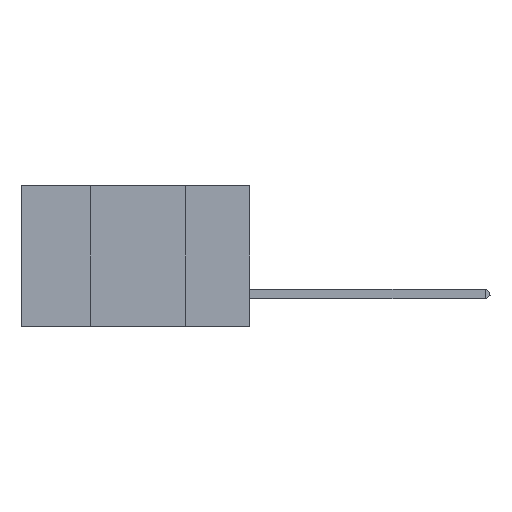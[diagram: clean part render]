
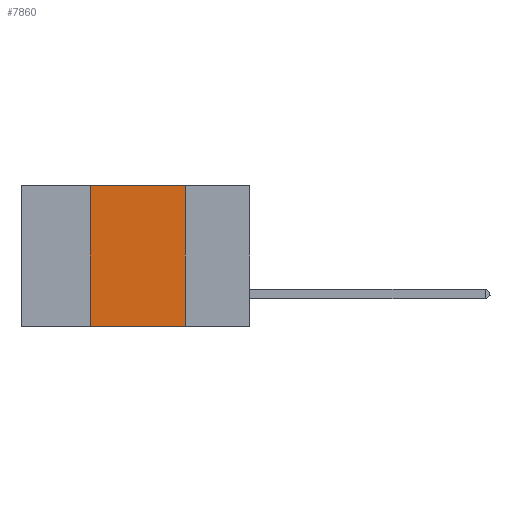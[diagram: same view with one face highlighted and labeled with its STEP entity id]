
A CAD part, left-side view. The second image highlights one B-rep face of the part: STEP entity #7860.
In plain terms, the highlighted planar face has unit normal (-1, 0, 0).
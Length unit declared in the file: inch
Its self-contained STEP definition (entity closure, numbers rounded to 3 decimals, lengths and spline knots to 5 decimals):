
#464 = CARTESIAN_POINT ( 'NONE',  ( 0., 0.42, 0. ) ) ;
#1630 = FACE_OUTER_BOUND ( 'NONE', #16072, .T. ) ;
#1831 = VERTEX_POINT ( 'NONE', #4936 ) ;
#2983 = LINE ( 'NONE', #19520, #17494 ) ;
#3559 = EDGE_CURVE ( 'NONE', #21737, #1831, #23307, .T. ) ;
#3567 = LINE ( 'NONE', #14143, #16220 ) ;
#3700 = DIRECTION ( 'NONE',  ( 0., 0., -1. ) ) ;
#4757 = DIRECTION ( 'NONE',  ( 1., 0., 0. ) ) ;
#4936 = CARTESIAN_POINT ( 'NONE',  ( 0., 0.17, -0.37 ) ) ;
#6666 = ORIENTED_EDGE ( 'NONE', *, *, #11246, .F. ) ;
#7860 = ADVANCED_FACE ( 'NONE', ( #1630 ), #10505, .F. ) ;
#7917 = DIRECTION ( 'NONE',  ( 0., 0., 1. ) ) ;
#8969 = CARTESIAN_POINT ( 'NONE',  ( 0., 0.17, 0. ) ) ;
#10505 = PLANE ( 'NONE',  #13052 ) ;
#11246 = EDGE_CURVE ( 'NONE', #14099, #21737, #2983, .T. ) ;
#11443 = VECTOR ( 'NONE', #7917, 39.37008 ) ;
#12001 = VERTEX_POINT ( 'NONE', #24842 ) ;
#12200 = EDGE_CURVE ( 'NONE', #12001, #14099, #16619, .T. ) ;
#12351 = DIRECTION ( 'NONE',  ( 0., -1., 0. ) ) ;
#12958 = ORIENTED_EDGE ( 'NONE', *, *, #3559, .F. ) ;
#13052 = AXIS2_PLACEMENT_3D ( 'NONE', #16476, #4757, #18497 ) ;
#14057 = EDGE_CURVE ( 'NONE', #12001, #1831, #3567, .T. ) ;
#14099 = VERTEX_POINT ( 'NONE', #464 ) ;
#14143 = CARTESIAN_POINT ( 'NONE',  ( 0., 0.6, -0.37 ) ) ;
#16072 = EDGE_LOOP ( 'NONE', ( #12958, #6666, #18748, #22351 ) ) ;
#16220 = VECTOR ( 'NONE', #12351, 39.37008 ) ;
#16476 = CARTESIAN_POINT ( 'NONE',  ( 0., 0.6, 0. ) ) ;
#16501 = VECTOR ( 'NONE', #3700, 39.37008 ) ;
#16619 = LINE ( 'NONE', #23509, #11443 ) ;
#17147 = CARTESIAN_POINT ( 'NONE',  ( 0., 0.17, 0. ) ) ;
#17334 = DIRECTION ( 'NONE',  ( 0., -1., 0. ) ) ;
#17494 = VECTOR ( 'NONE', #17334, 39.37008 ) ;
#18497 = DIRECTION ( 'NONE',  ( 0., 0., -1. ) ) ;
#18748 = ORIENTED_EDGE ( 'NONE', *, *, #12200, .F. ) ;
#19520 = CARTESIAN_POINT ( 'NONE',  ( 0., 0.6, 0. ) ) ;
#21737 = VERTEX_POINT ( 'NONE', #8969 ) ;
#22351 = ORIENTED_EDGE ( 'NONE', *, *, #14057, .T. ) ;
#23307 = LINE ( 'NONE', #17147, #16501 ) ;
#23509 = CARTESIAN_POINT ( 'NONE',  ( 0., 0.42, 0. ) ) ;
#24842 = CARTESIAN_POINT ( 'NONE',  ( 0., 0.42, -0.37 ) ) ;
